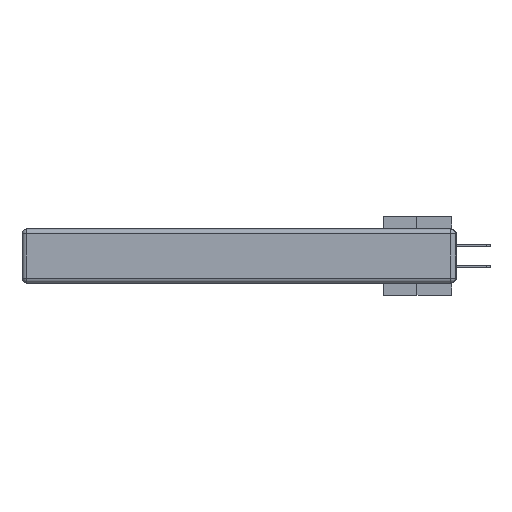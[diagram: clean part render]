
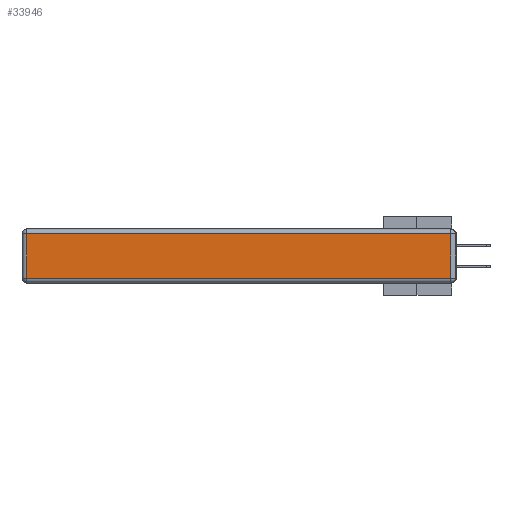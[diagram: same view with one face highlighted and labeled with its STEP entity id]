
A CAD part, left-side view. The second image highlights one B-rep face of the part: STEP entity #33946.
In plain terms, the highlighted planar face has unit normal (-1, 0, 0).
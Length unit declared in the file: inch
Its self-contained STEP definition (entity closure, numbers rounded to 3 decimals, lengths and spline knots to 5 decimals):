
#1323 = EDGE_CURVE ( 'NONE', #26584, #12407, #8277, .T. ) ;
#1567 = CARTESIAN_POINT ( 'NONE',  ( 0., 0.03, -0.313 ) ) ;
#1682 = AXIS2_PLACEMENT_3D ( 'NONE', #34796, #26135, #11969 ) ;
#4147 = LINE ( 'NONE', #7624, #27089 ) ;
#5913 = EDGE_LOOP ( 'NONE', ( #17898, #27922, #18388, #24039 ) ) ;
#6084 = VECTOR ( 'NONE', #32940, 39.37008 ) ;
#7624 = CARTESIAN_POINT ( 'NONE',  ( 0., 2.75, -0.03 ) ) ;
#8189 = LINE ( 'NONE', #18112, #25001 ) ;
#8239 = VECTOR ( 'NONE', #22176, 39.37008 ) ;
#8277 = LINE ( 'NONE', #24414, #6084 ) ;
#11969 = DIRECTION ( 'NONE',  ( 0., 0., 1. ) ) ;
#12407 = VERTEX_POINT ( 'NONE', #33473 ) ;
#12895 = VERTEX_POINT ( 'NONE', #23698 ) ;
#12998 = EDGE_CURVE ( 'NONE', #12407, #12895, #4147, .T. ) ;
#17898 = ORIENTED_EDGE ( 'NONE', *, *, #35620, .T. ) ;
#18112 = CARTESIAN_POINT ( 'NONE',  ( 0., 2.72, -0.343 ) ) ;
#18388 = ORIENTED_EDGE ( 'NONE', *, *, #12998, .T. ) ;
#19822 = VERTEX_POINT ( 'NONE', #31279 ) ;
#20605 = PLANE ( 'NONE',  #1682 ) ;
#20942 = DIRECTION ( 'NONE',  ( 0., 0., -1. ) ) ;
#22176 = DIRECTION ( 'NONE',  ( 0., -1., 0. ) ) ;
#23698 = CARTESIAN_POINT ( 'NONE',  ( 0., 2.72, -0.03 ) ) ;
#24039 = ORIENTED_EDGE ( 'NONE', *, *, #28489, .T. ) ;
#24414 = CARTESIAN_POINT ( 'NONE',  ( 0., 0.03, -0.343 ) ) ;
#24748 = FACE_OUTER_BOUND ( 'NONE', #5913, .T. ) ;
#25001 = VECTOR ( 'NONE', #20942, 39.37008 ) ;
#25474 = LINE ( 'NONE', #28329, #8239 ) ;
#26135 = DIRECTION ( 'NONE',  ( -1., 0., 0. ) ) ;
#26584 = VERTEX_POINT ( 'NONE', #1567 ) ;
#27089 = VECTOR ( 'NONE', #32821, 39.37008 ) ;
#27922 = ORIENTED_EDGE ( 'NONE', *, *, #1323, .T. ) ;
#28329 = CARTESIAN_POINT ( 'NONE',  ( 0., 0., -0.313 ) ) ;
#28489 = EDGE_CURVE ( 'NONE', #12895, #19822, #8189, .T. ) ;
#31279 = CARTESIAN_POINT ( 'NONE',  ( 0., 2.72, -0.313 ) ) ;
#32821 = DIRECTION ( 'NONE',  ( 0., 1., 0. ) ) ;
#32940 = DIRECTION ( 'NONE',  ( 0., 0., 1. ) ) ;
#33473 = CARTESIAN_POINT ( 'NONE',  ( 0., 0.03, -0.03 ) ) ;
#33946 = ADVANCED_FACE ( 'NONE', ( #24748 ), #20605, .T. ) ;
#34796 = CARTESIAN_POINT ( 'NONE',  ( 0., 0., -0.343 ) ) ;
#35620 = EDGE_CURVE ( 'NONE', #19822, #26584, #25474, .T. ) ;
